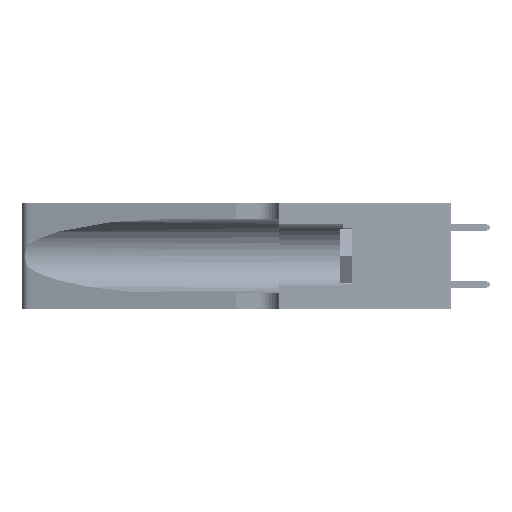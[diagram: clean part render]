
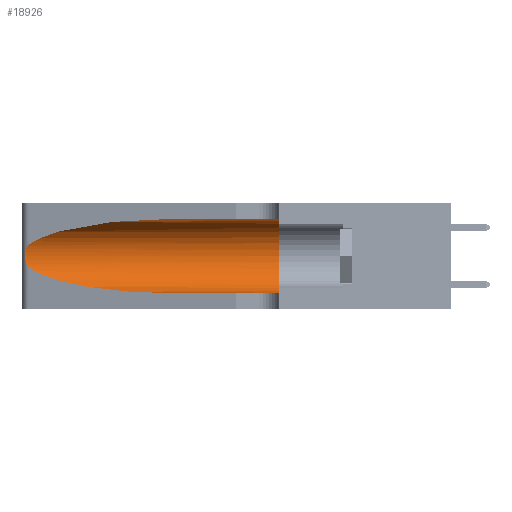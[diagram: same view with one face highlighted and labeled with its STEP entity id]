
A CAD part, left-side view. The second image highlights one B-rep face of the part: STEP entity #18926.
In plain terms, the highlighted cylindrical face has radius 3.308 mm (diameter 6.617 mm), a partial arc.
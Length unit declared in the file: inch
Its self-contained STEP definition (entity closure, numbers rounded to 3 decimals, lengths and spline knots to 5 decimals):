
#223 = VECTOR ( 'NONE', #41311, 39.37008 ) ;
#647 = CARTESIAN_POINT ( 'NONE',  ( 0.1305, 0.72297, 0.31525 ) ) ;
#2194 = B_SPLINE_CURVE_WITH_KNOTS ( 'NONE', 3,
 ( #44936, #49093, #20231, #53213, #28505, #3905, #32651, #8014, #36840, #12100, #41000, #16272, #45105, #20403 ),
 .UNSPECIFIED., .F., .F.,
 ( 4, 2, 2, 2, 2, 2, 4 ),
 ( 0., 0.00027, 0.00053, 0.00107, 0.0016, 0.00187, 0.00214 ),
 .UNSPECIFIED. ) ;
#2909 = DIRECTION ( 'NONE',  ( 0., 0., 1. ) ) ;
#3905 = CARTESIAN_POINT ( 'NONE',  ( 0.26018, 1.23835, 0.19895 ) ) ;
#4623 = CARTESIAN_POINT ( 'NONE',  ( 0.2373, 1.15595, 0.08982 ) ) ;
#4992 = CYLINDRICAL_SURFACE ( 'NONE', #36928, 0.13025 ) ;
#5551 = CARTESIAN_POINT ( 'NONE',  ( 0.2373, 1.15595, 0.28018 ) ) ;
#8014 = CARTESIAN_POINT ( 'NONE',  ( 0.26075, 1.23896, 0.178 ) ) ;
#9997 = ORIENTED_EDGE ( 'NONE', *, *, #24792, .F. ) ;
#10291 = LINE ( 'NONE', #37318, #39318 ) ;
#10512 = VERTEX_POINT ( 'NONE', #647 ) ;
#11168 = LINE ( 'NONE', #12253, #223 ) ;
#11633 = CARTESIAN_POINT ( 'NONE',  ( 0.1305, 1.61858, 0.185 ) ) ;
#12100 = CARTESIAN_POINT ( 'NONE',  ( 0.25856, 1.23593, 0.16098 ) ) ;
#12253 = CARTESIAN_POINT ( 'NONE',  ( 0.1305, 1.61858, 0.31525 ) ) ;
#12842 = CARTESIAN_POINT ( 'NONE',  ( 0.18966, 0.96281, 0.05475 ) ) ;
#12949 = EDGE_CURVE ( 'NONE', #36828, #38107, #2194, .T. ) ;
#13678 = CARTESIAN_POINT ( 'NONE',  ( 0.25487, 1.22718, 0.14631 ) ) ;
#15112 = ORIENTED_EDGE ( 'NONE', *, *, #28021, .T. ) ;
#15803 = VERTEX_POINT ( 'NONE', #34011 ) ;
#16272 = CARTESIAN_POINT ( 'NONE',  ( 0.25639, 1.23186, 0.15144 ) ) ;
#16548 =( BOUNDED_CURVE ( )  B_SPLINE_CURVE ( 3, ( #33360, #4623, #12842, #41716 ),
 .UNSPECIFIED., .F., .F. ) 
 B_SPLINE_CURVE_WITH_KNOTS ( ( 4, 4 ),
 ( 3.44316, 4.71239 ),
 .UNSPECIFIED. ) 
 CURVE ( )  GEOMETRIC_REPRESENTATION_ITEM ( )  RATIONAL_B_SPLINE_CURVE ( ( 1., 0.87, 0.87, 1. ) ) 
 REPRESENTATION_ITEM ( '' )  );
#16760 = DIRECTION ( 'NONE',  ( 0., -1., 0. ) ) ;
#17620 = EDGE_LOOP ( 'NONE', ( #27986, #22188, #15112, #33824, #28029, #9997 ) ) ;
#18819 = CARTESIAN_POINT ( 'NONE',  ( 0.1305, 0.72297, 0.05475 ) ) ;
#18926 = ADVANCED_FACE ( 'NONE', ( #28142 ), #4992, .F. ) ;
#20231 = CARTESIAN_POINT ( 'NONE',  ( 0.25639, 1.23184, 0.21858 ) ) ;
#20403 = CARTESIAN_POINT ( 'NONE',  ( 0.25487, 1.22718, 0.14631 ) ) ;
#20447 = EDGE_CURVE ( 'NONE', #10512, #36828, #47604, .T. ) ;
#22188 = ORIENTED_EDGE ( 'NONE', *, *, #12949, .T. ) ;
#24009 = VERTEX_POINT ( 'NONE', #18819 ) ;
#24792 = EDGE_CURVE ( 'NONE', #10512, #15803, #11168, .T. ) ;
#25257 = EDGE_CURVE ( 'NONE', #15803, #31715, #52398, .T. ) ;
#26006 = CARTESIAN_POINT ( 'NONE',  ( 0.1305, 0.72297, 0.31525 ) ) ;
#27514 = DIRECTION ( 'NONE',  ( 0., 1., 0. ) ) ;
#27986 = ORIENTED_EDGE ( 'NONE', *, *, #20447, .T. ) ;
#28021 = EDGE_CURVE ( 'NONE', #38107, #24009, #16548, .T. ) ;
#28029 = ORIENTED_EDGE ( 'NONE', *, *, #25257, .F. ) ;
#28142 = FACE_OUTER_BOUND ( 'NONE', #17620, .T. ) ;
#28505 = CARTESIAN_POINT ( 'NONE',  ( 0.25854, 1.2359, 0.20912 ) ) ;
#29194 = CARTESIAN_POINT ( 'NONE',  ( 0.25487, 1.22718, 0.22369 ) ) ;
#31715 = VERTEX_POINT ( 'NONE', #32149 ) ;
#32149 = CARTESIAN_POINT ( 'NONE',  ( 0.1305, 0.35, 0.05475 ) ) ;
#32651 = CARTESIAN_POINT ( 'NONE',  ( 0.26075, 1.23896, 0.19203 ) ) ;
#33360 = CARTESIAN_POINT ( 'NONE',  ( 0.25487, 1.22718, 0.14631 ) ) ;
#33824 = ORIENTED_EDGE ( 'NONE', *, *, #37920, .T. ) ;
#34011 = CARTESIAN_POINT ( 'NONE',  ( 0.1305, 0.35, 0.31525 ) ) ;
#34306 = CARTESIAN_POINT ( 'NONE',  ( 0.25487, 1.22718, 0.22369 ) ) ;
#36714 = AXIS2_PLACEMENT_3D ( 'NONE', #52233, #27514, #2909 ) ;
#36828 = VERTEX_POINT ( 'NONE', #29194 ) ;
#36840 = CARTESIAN_POINT ( 'NONE',  ( 0.26017, 1.23833, 0.17102 ) ) ;
#36928 = AXIS2_PLACEMENT_3D ( 'NONE', #11633, #48752, #52917 ) ;
#37318 = CARTESIAN_POINT ( 'NONE',  ( 0.1305, 1.61858, 0.05475 ) ) ;
#37920 = EDGE_CURVE ( 'NONE', #24009, #31715, #10291, .T. ) ;
#38107 = VERTEX_POINT ( 'NONE', #13678 ) ;
#39318 = VECTOR ( 'NONE', #16760, 39.37008 ) ;
#41000 = CARTESIAN_POINT ( 'NONE',  ( 0.25789, 1.23486, 0.15765 ) ) ;
#41311 = DIRECTION ( 'NONE',  ( 0., -1., 0. ) ) ;
#41716 = CARTESIAN_POINT ( 'NONE',  ( 0.1305, 0.72297, 0.05475 ) ) ;
#44936 = CARTESIAN_POINT ( 'NONE',  ( 0.25487, 1.22718, 0.22369 ) ) ;
#45105 = CARTESIAN_POINT ( 'NONE',  ( 0.25555, 1.22993, 0.14849 ) ) ;
#47604 =( BOUNDED_CURVE ( )  B_SPLINE_CURVE ( 3, ( #26006, #50725, #5551, #34306 ),
 .UNSPECIFIED., .F., .F. ) 
 B_SPLINE_CURVE_WITH_KNOTS ( ( 4, 4 ),
 ( 1.5708, 2.84003 ),
 .UNSPECIFIED. ) 
 CURVE ( )  GEOMETRIC_REPRESENTATION_ITEM ( )  RATIONAL_B_SPLINE_CURVE ( ( 1., 0.87, 0.87, 1. ) ) 
 REPRESENTATION_ITEM ( '' )  );
#48752 = DIRECTION ( 'NONE',  ( 0., -1., 0. ) ) ;
#49093 = CARTESIAN_POINT ( 'NONE',  ( 0.25555, 1.22994, 0.2215 ) ) ;
#50725 = CARTESIAN_POINT ( 'NONE',  ( 0.18966, 0.96281, 0.31525 ) ) ;
#52233 = CARTESIAN_POINT ( 'NONE',  ( 0.1305, 0.35, 0.185 ) ) ;
#52398 = CIRCLE ( 'NONE', #36714, 0.13025 ) ;
#52917 = DIRECTION ( 'NONE',  ( 0., 0., -1. ) ) ;
#53213 = CARTESIAN_POINT ( 'NONE',  ( 0.25787, 1.23484, 0.2124 ) ) ;
